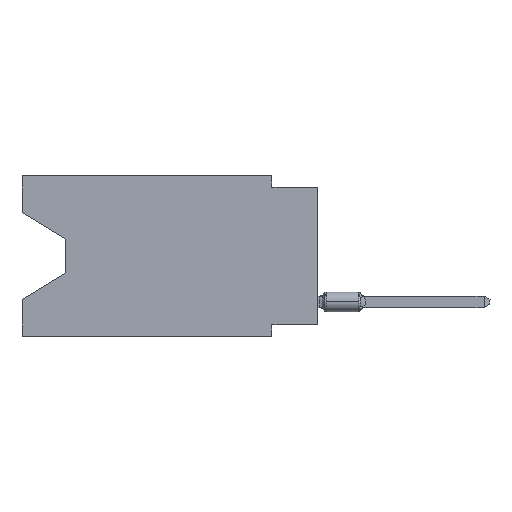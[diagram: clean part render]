
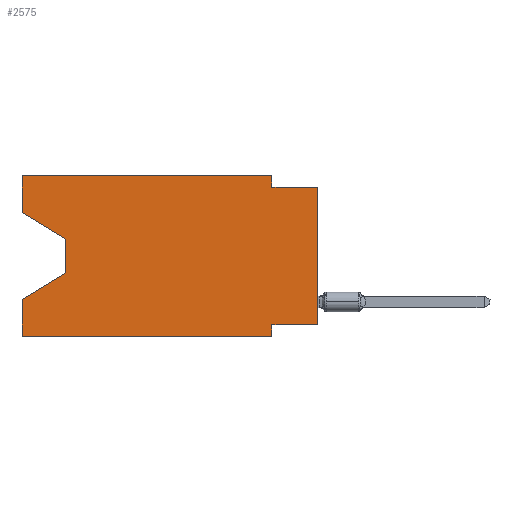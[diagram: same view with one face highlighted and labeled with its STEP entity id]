
A CAD part, left-side view. The second image highlights one B-rep face of the part: STEP entity #2575.
In plain terms, the highlighted planar face has unit normal (-1, 0, 0).
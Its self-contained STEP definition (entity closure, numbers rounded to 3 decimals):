
#177 = ORIENTED_EDGE ( 'NONE', *, *, #1340, .T. ) ;
#207 = CARTESIAN_POINT ( 'NONE',  ( 0., 13.97, -5.385 ) ) ;
#269 = LINE ( 'NONE', #10516, #5433 ) ;
#382 = VERTEX_POINT ( 'NONE', #8849 ) ;
#403 = VECTOR ( 'NONE', #8419, 1000. ) ;
#443 = VECTOR ( 'NONE', #2339, 1000. ) ;
#598 = DIRECTION ( 'NONE',  ( 0., 0., -1. ) ) ;
#605 = EDGE_CURVE ( 'NONE', #15437, #16238, #3371, .T. ) ;
#691 = DIRECTION ( 'NONE',  ( 0., 0., 1. ) ) ;
#966 = EDGE_CURVE ( 'NONE', #9930, #10202, #15934, .T. ) ;
#1340 = EDGE_CURVE ( 'NONE', #8702, #16238, #10296, .T. ) ;
#1518 = DIRECTION ( 'NONE',  ( 0., 0., -1. ) ) ;
#1598 = LINE ( 'NONE', #15256, #3049 ) ;
#1775 = CARTESIAN_POINT ( 'NONE',  ( 0., 0., -8.255 ) ) ;
#1869 = CARTESIAN_POINT ( 'NONE',  ( 0., 0., -8.255 ) ) ;
#2026 = DIRECTION ( 'NONE',  ( 0., 0., 1. ) ) ;
#2028 = CARTESIAN_POINT ( 'NONE',  ( 0., 16.383, 0. ) ) ;
#2339 = DIRECTION ( 'NONE',  ( 0., 0., -1. ) ) ;
#2492 = VERTEX_POINT ( 'NONE', #207 ) ;
#2575 = ADVANCED_FACE ( 'NONE', ( #11932 ), #4570, .F. ) ;
#2834 = VECTOR ( 'NONE', #2026, 1000. ) ;
#2851 = CARTESIAN_POINT ( 'NONE',  ( 0., 0., 0. ) ) ;
#3011 = DIRECTION ( 'NONE',  ( 0., -1., 0. ) ) ;
#3049 = VECTOR ( 'NONE', #1518, 1000. ) ;
#3251 = CARTESIAN_POINT ( 'NONE',  ( 0., 16.383, -8.89 ) ) ;
#3371 = LINE ( 'NONE', #10722, #403 ) ;
#3957 = LINE ( 'NONE', #1775, #10538 ) ;
#4397 = VECTOR ( 'NONE', #3011, 1000. ) ;
#4570 = PLANE ( 'NONE',  #14067 ) ;
#4596 = EDGE_CURVE ( 'NONE', #5082, #382, #8992, .T. ) ;
#4643 = VERTEX_POINT ( 'NONE', #6742 ) ;
#4758 = CARTESIAN_POINT ( 'NONE',  ( 0., 16.383, -2.038 ) ) ;
#5082 = VERTEX_POINT ( 'NONE', #8972 ) ;
#5191 = CARTESIAN_POINT ( 'NONE',  ( 0., 16.383, -8.89 ) ) ;
#5433 = VECTOR ( 'NONE', #11752, 1000. ) ;
#5468 = ORIENTED_EDGE ( 'NONE', *, *, #4596, .F. ) ;
#5754 = CARTESIAN_POINT ( 'NONE',  ( 0., 16.383, 0. ) ) ;
#5811 = ORIENTED_EDGE ( 'NONE', *, *, #10432, .T. ) ;
#5821 = EDGE_CURVE ( 'NONE', #8702, #5082, #3957, .T. ) ;
#6075 = ORIENTED_EDGE ( 'NONE', *, *, #13909, .T. ) ;
#6568 = VECTOR ( 'NONE', #13117, 1000. ) ;
#6659 = CARTESIAN_POINT ( 'NONE',  ( 0., 0., -0.635 ) ) ;
#6742 = CARTESIAN_POINT ( 'NONE',  ( 0., 13.97, -3.505 ) ) ;
#6781 = ORIENTED_EDGE ( 'NONE', *, *, #966, .F. ) ;
#6825 = LINE ( 'NONE', #3251, #4397 ) ;
#7155 = ORIENTED_EDGE ( 'NONE', *, *, #10183, .F. ) ;
#7230 = CARTESIAN_POINT ( 'NONE',  ( 0., 16.383, 0. ) ) ;
#7244 = LINE ( 'NONE', #4758, #10979 ) ;
#7336 = CARTESIAN_POINT ( 'NONE',  ( 0., 2.54, -8.89 ) ) ;
#7858 = VERTEX_POINT ( 'NONE', #12229 ) ;
#7960 = ORIENTED_EDGE ( 'NONE', *, *, #9037, .T. ) ;
#8076 = LINE ( 'NONE', #2028, #6568 ) ;
#8386 = DIRECTION ( 'NONE',  ( 1., 0., 0. ) ) ;
#8393 = LINE ( 'NONE', #16000, #10177 ) ;
#8405 = DIRECTION ( 'NONE',  ( 0., -0.855, -0.519 ) ) ;
#8419 = DIRECTION ( 'NONE',  ( 0., -1., 0. ) ) ;
#8702 = VERTEX_POINT ( 'NONE', #1869 ) ;
#8849 = CARTESIAN_POINT ( 'NONE',  ( 0., 2.54, -8.89 ) ) ;
#8972 = CARTESIAN_POINT ( 'NONE',  ( 0., 2.54, -8.255 ) ) ;
#8992 = LINE ( 'NONE', #7336, #13960 ) ;
#9037 = EDGE_CURVE ( 'NONE', #11130, #382, #6825, .T. ) ;
#9628 = VERTEX_POINT ( 'NONE', #10077 ) ;
#9855 = CARTESIAN_POINT ( 'NONE',  ( 0., 2.54, -0.635 ) ) ;
#9930 = VERTEX_POINT ( 'NONE', #12199 ) ;
#9941 = CARTESIAN_POINT ( 'NONE',  ( 0., 13.97, -3.505 ) ) ;
#10077 = CARTESIAN_POINT ( 'NONE',  ( 0., 16.383, -6.852 ) ) ;
#10177 = VECTOR ( 'NONE', #691, 1000. ) ;
#10183 = EDGE_CURVE ( 'NONE', #11130, #9628, #8393, .T. ) ;
#10202 = VERTEX_POINT ( 'NONE', #7230 ) ;
#10296 = LINE ( 'NONE', #2851, #11701 ) ;
#10432 = EDGE_CURVE ( 'NONE', #2492, #9628, #269, .T. ) ;
#10516 = CARTESIAN_POINT ( 'NONE',  ( 0., 13.97, -5.385 ) ) ;
#10534 = EDGE_CURVE ( 'NONE', #7858, #15437, #1598, .T. ) ;
#10538 = VECTOR ( 'NONE', #14050, 1000. ) ;
#10594 = ORIENTED_EDGE ( 'NONE', *, *, #10534, .F. ) ;
#10722 = CARTESIAN_POINT ( 'NONE',  ( 0., 0., -0.635 ) ) ;
#10979 = VECTOR ( 'NONE', #8405, 1000. ) ;
#11014 = CARTESIAN_POINT ( 'NONE',  ( 0., 16.383, 0. ) ) ;
#11130 = VERTEX_POINT ( 'NONE', #5191 ) ;
#11701 = VECTOR ( 'NONE', #15347, 1000. ) ;
#11752 = DIRECTION ( 'NONE',  ( 0., 0.855, -0.519 ) ) ;
#11932 = FACE_OUTER_BOUND ( 'NONE', #14072, .T. ) ;
#12199 = CARTESIAN_POINT ( 'NONE',  ( 0., 16.383, -2.038 ) ) ;
#12229 = CARTESIAN_POINT ( 'NONE',  ( 0., 2.54, 0. ) ) ;
#12364 = DIRECTION ( 'NONE',  ( 0., 0., -1. ) ) ;
#12825 = ORIENTED_EDGE ( 'NONE', *, *, #16120, .F. ) ;
#13117 = DIRECTION ( 'NONE',  ( 0., -1., 0. ) ) ;
#13747 = ORIENTED_EDGE ( 'NONE', *, *, #5821, .F. ) ;
#13756 = LINE ( 'NONE', #9941, #443 ) ;
#13909 = EDGE_CURVE ( 'NONE', #9930, #4643, #7244, .T. ) ;
#13960 = VECTOR ( 'NONE', #12364, 1000. ) ;
#14050 = DIRECTION ( 'NONE',  ( 0., 1., 0. ) ) ;
#14067 = AXIS2_PLACEMENT_3D ( 'NONE', #11014, #8386, #598 ) ;
#14072 = EDGE_LOOP ( 'NONE', ( #6075, #16272, #5811, #7155, #7960, #5468, #13747, #177, #15885, #10594, #12825, #6781 ) ) ;
#14446 = EDGE_CURVE ( 'NONE', #4643, #2492, #13756, .T. ) ;
#15256 = CARTESIAN_POINT ( 'NONE',  ( 0., 2.54, 0. ) ) ;
#15347 = DIRECTION ( 'NONE',  ( 0., 0., 1. ) ) ;
#15437 = VERTEX_POINT ( 'NONE', #9855 ) ;
#15885 = ORIENTED_EDGE ( 'NONE', *, *, #605, .F. ) ;
#15934 = LINE ( 'NONE', #5754, #2834 ) ;
#16000 = CARTESIAN_POINT ( 'NONE',  ( 0., 16.383, 0. ) ) ;
#16120 = EDGE_CURVE ( 'NONE', #10202, #7858, #8076, .T. ) ;
#16238 = VERTEX_POINT ( 'NONE', #6659 ) ;
#16272 = ORIENTED_EDGE ( 'NONE', *, *, #14446, .T. ) ;
